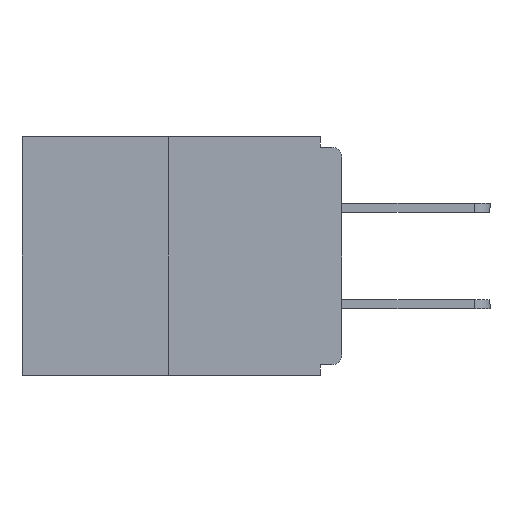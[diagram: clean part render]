
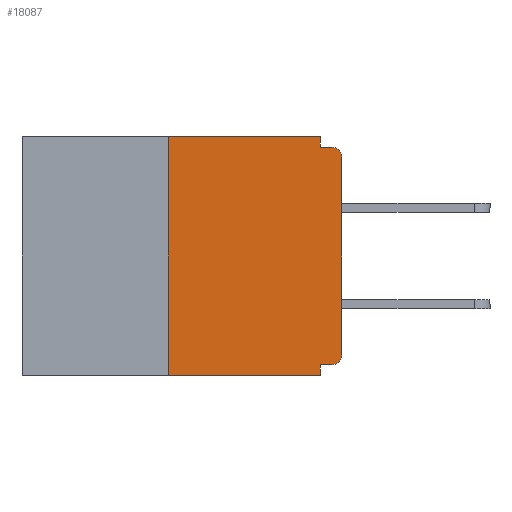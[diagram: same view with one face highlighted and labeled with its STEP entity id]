
A CAD part, left-side view. The second image highlights one B-rep face of the part: STEP entity #18087.
In plain terms, the highlighted planar face has unit normal (-1, 0, 0).
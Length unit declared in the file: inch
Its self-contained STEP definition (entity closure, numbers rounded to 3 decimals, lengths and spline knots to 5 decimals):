
#151 = AXIS2_PLACEMENT_3D ( 'NONE', #19039, #23228, #12782 ) ;
#183 = DIRECTION ( 'NONE',  ( -1., 0., 0. ) ) ;
#551 = DIRECTION ( 'NONE',  ( 0., 0., -1. ) ) ;
#1586 = VECTOR ( 'NONE', #12267, 39.37008 ) ;
#1812 = CARTESIAN_POINT ( 'NONE',  ( 0., 0.031, -0.343 ) ) ;
#1919 = ORIENTED_EDGE ( 'NONE', *, *, #11049, .F. ) ;
#1978 = DIRECTION ( 'NONE',  ( 0., 0., 1. ) ) ;
#2033 = CARTESIAN_POINT ( 'NONE',  ( 0., 0.031, 0. ) ) ;
#2215 = ORIENTED_EDGE ( 'NONE', *, *, #8458, .F. ) ;
#2555 = CARTESIAN_POINT ( 'NONE',  ( 0., 0.031, -0.328 ) ) ;
#2708 = LINE ( 'NONE', #4547, #22208 ) ;
#2864 = CARTESIAN_POINT ( 'NONE',  ( 0., 0., 0. ) ) ;
#2897 = CARTESIAN_POINT ( 'NONE',  ( 0., 0.46, 0. ) ) ;
#3050 = ORIENTED_EDGE ( 'NONE', *, *, #26210, .F. ) ;
#3384 = AXIS2_PLACEMENT_3D ( 'NONE', #9237, #15199, #551 ) ;
#3920 = VERTEX_POINT ( 'NONE', #5887 ) ;
#4107 = LINE ( 'NONE', #1812, #25564 ) ;
#4211 = ORIENTED_EDGE ( 'NONE', *, *, #9034, .F. ) ;
#4275 = DIRECTION ( 'NONE',  ( 0., 0., -1. ) ) ;
#4547 = CARTESIAN_POINT ( 'NONE',  ( 0., 0.46, -0.343 ) ) ;
#5189 = LINE ( 'NONE', #19823, #8145 ) ;
#5703 = CARTESIAN_POINT ( 'NONE',  ( 0., 0., -0.03 ) ) ;
#5736 = VERTEX_POINT ( 'NONE', #12918 ) ;
#5887 = CARTESIAN_POINT ( 'NONE',  ( 0., 0.015, -0.328 ) ) ;
#6000 = VERTEX_POINT ( 'NONE', #5703 ) ;
#6718 = ORIENTED_EDGE ( 'NONE', *, *, #24725, .T. ) ;
#6846 = EDGE_CURVE ( 'NONE', #20446, #5736, #18374, .T. ) ;
#7162 = VECTOR ( 'NONE', #1978, 39.37008 ) ;
#7883 = EDGE_LOOP ( 'NONE', ( #15880, #27123, #14329, #2215, #3050, #6718, #16876, #10181, #1919, #4211 ) ) ;
#8145 = VECTOR ( 'NONE', #22070, 39.37008 ) ;
#8439 = PLANE ( 'NONE',  #151 ) ;
#8458 = EDGE_CURVE ( 'NONE', #25319, #9336, #4107, .T. ) ;
#9034 = EDGE_CURVE ( 'NONE', #20535, #14522, #14581, .T. ) ;
#9237 = CARTESIAN_POINT ( 'NONE',  ( 0., 0.015, -0.313 ) ) ;
#9336 = VERTEX_POINT ( 'NONE', #15908 ) ;
#9971 = VECTOR ( 'NONE', #25097, 39.37008 ) ;
#10181 = ORIENTED_EDGE ( 'NONE', *, *, #22555, .T. ) ;
#11049 = EDGE_CURVE ( 'NONE', #14522, #14309, #5189, .T. ) ;
#11322 = VECTOR ( 'NONE', #23864, 39.37008 ) ;
#11522 = FACE_OUTER_BOUND ( 'NONE', #7883, .T. ) ;
#12267 = DIRECTION ( 'NONE',  ( 0., 0., 1. ) ) ;
#12764 = DIRECTION ( 'NONE',  ( 0., 0., -1. ) ) ;
#12782 = DIRECTION ( 'NONE',  ( 0., 0., -1. ) ) ;
#12918 = CARTESIAN_POINT ( 'NONE',  ( 0., 0.25, 0. ) ) ;
#13270 = CARTESIAN_POINT ( 'NONE',  ( 0., 0.015, -0.015 ) ) ;
#13582 = LINE ( 'NONE', #24819, #9971 ) ;
#13934 = VECTOR ( 'NONE', #18596, 39.37008 ) ;
#14106 = VERTEX_POINT ( 'NONE', #23756 ) ;
#14309 = VERTEX_POINT ( 'NONE', #13270 ) ;
#14329 = ORIENTED_EDGE ( 'NONE', *, *, #25813, .T. ) ;
#14522 = VERTEX_POINT ( 'NONE', #18873 ) ;
#14581 = LINE ( 'NONE', #16706, #13934 ) ;
#15199 = DIRECTION ( 'NONE',  ( -1., 0., 0. ) ) ;
#15880 = ORIENTED_EDGE ( 'NONE', *, *, #16037, .F. ) ;
#15908 = CARTESIAN_POINT ( 'NONE',  ( 0., 0.031, -0.343 ) ) ;
#16037 = EDGE_CURVE ( 'NONE', #5736, #20535, #24197, .T. ) ;
#16706 = CARTESIAN_POINT ( 'NONE',  ( 0., 0.031, 0. ) ) ;
#16876 = ORIENTED_EDGE ( 'NONE', *, *, #17783, .T. ) ;
#16942 = CARTESIAN_POINT ( 'NONE',  ( 0., 0.015, -0.03 ) ) ;
#17033 = CIRCLE ( 'NONE', #23798, 0.015 ) ;
#17783 = EDGE_CURVE ( 'NONE', #14106, #6000, #25738, .T. ) ;
#18087 = ADVANCED_FACE ( 'NONE', ( #11522 ), #8439, .F. ) ;
#18374 = LINE ( 'NONE', #23243, #7162 ) ;
#18596 = DIRECTION ( 'NONE',  ( 0., 0., -1. ) ) ;
#18740 = CARTESIAN_POINT ( 'NONE',  ( 0., 0.25, -0.343 ) ) ;
#18873 = CARTESIAN_POINT ( 'NONE',  ( 0., 0.031, -0.015 ) ) ;
#19039 = CARTESIAN_POINT ( 'NONE',  ( 0., 0.46, 0. ) ) ;
#19278 = DIRECTION ( 'NONE',  ( 0., -1., 0. ) ) ;
#19823 = CARTESIAN_POINT ( 'NONE',  ( 0., 0., -0.015 ) ) ;
#20446 = VERTEX_POINT ( 'NONE', #18740 ) ;
#20535 = VERTEX_POINT ( 'NONE', #2033 ) ;
#22070 = DIRECTION ( 'NONE',  ( 0., -1., 0. ) ) ;
#22208 = VECTOR ( 'NONE', #19278, 39.37008 ) ;
#22555 = EDGE_CURVE ( 'NONE', #6000, #14309, #17033, .T. ) ;
#23228 = DIRECTION ( 'NONE',  ( 1., 0., 0. ) ) ;
#23243 = CARTESIAN_POINT ( 'NONE',  ( 0., 0.25, 0. ) ) ;
#23756 = CARTESIAN_POINT ( 'NONE',  ( 0., 0., -0.313 ) ) ;
#23798 = AXIS2_PLACEMENT_3D ( 'NONE', #16942, #183, #4275 ) ;
#23864 = DIRECTION ( 'NONE',  ( 0., -1., 0. ) ) ;
#24197 = LINE ( 'NONE', #2897, #11322 ) ;
#24725 = EDGE_CURVE ( 'NONE', #3920, #14106, #26236, .T. ) ;
#24819 = CARTESIAN_POINT ( 'NONE',  ( 0., 0., -0.328 ) ) ;
#25097 = DIRECTION ( 'NONE',  ( 0., 1., 0. ) ) ;
#25319 = VERTEX_POINT ( 'NONE', #2555 ) ;
#25564 = VECTOR ( 'NONE', #12764, 39.37008 ) ;
#25738 = LINE ( 'NONE', #2864, #1586 ) ;
#25813 = EDGE_CURVE ( 'NONE', #20446, #9336, #2708, .T. ) ;
#26210 = EDGE_CURVE ( 'NONE', #3920, #25319, #13582, .T. ) ;
#26236 = CIRCLE ( 'NONE', #3384, 0.015 ) ;
#27123 = ORIENTED_EDGE ( 'NONE', *, *, #6846, .F. ) ;
